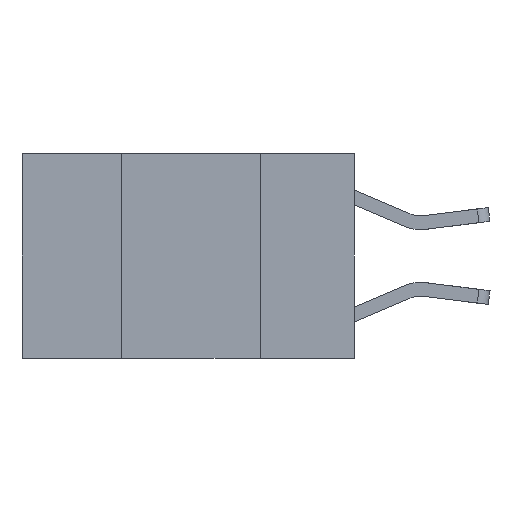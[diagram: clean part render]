
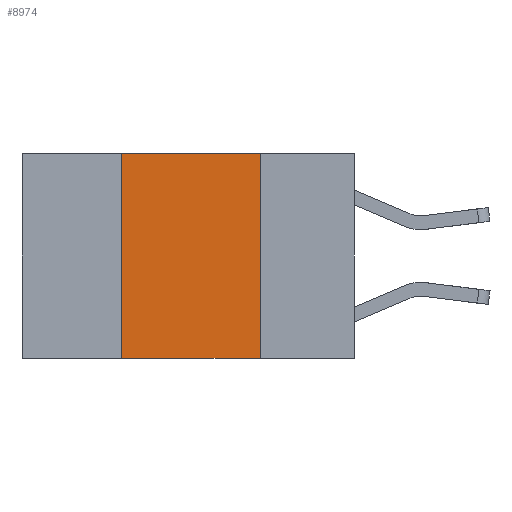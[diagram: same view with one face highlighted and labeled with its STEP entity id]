
A CAD part, left-side view. The second image highlights one B-rep face of the part: STEP entity #8974.
In plain terms, the highlighted planar face has unit normal (-1, 0, 0).
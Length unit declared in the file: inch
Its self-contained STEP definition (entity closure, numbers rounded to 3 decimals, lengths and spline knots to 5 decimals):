
#59 = VERTEX_POINT ( 'NONE', #8099 ) ;
#444 = CARTESIAN_POINT ( 'NONE',  ( 0., 0.42, 0. ) ) ;
#585 = EDGE_LOOP ( 'NONE', ( #4037, #6360, #8165, #7606 ) ) ;
#648 = LINE ( 'NONE', #1263, #4809 ) ;
#688 = DIRECTION ( 'NONE',  ( 0., -1., 0. ) ) ;
#1263 = CARTESIAN_POINT ( 'NONE',  ( 0., 0.17, 0. ) ) ;
#1276 = DIRECTION ( 'NONE',  ( 0., 0., -1. ) ) ;
#1296 = EDGE_CURVE ( 'NONE', #3190, #59, #648, .T. ) ;
#1344 = VERTEX_POINT ( 'NONE', #444 ) ;
#1619 = DIRECTION ( 'NONE',  ( 0., 0., 1. ) ) ;
#1663 = DIRECTION ( 'NONE',  ( 1., 0., 0. ) ) ;
#2662 = LINE ( 'NONE', #5832, #8879 ) ;
#3190 = VERTEX_POINT ( 'NONE', #5365 ) ;
#3290 = CARTESIAN_POINT ( 'NONE',  ( 0., 0.42, 0. ) ) ;
#4037 = ORIENTED_EDGE ( 'NONE', *, *, #1296, .F. ) ;
#4129 = PLANE ( 'NONE',  #4927 ) ;
#4809 = VECTOR ( 'NONE', #1276, 39.37008 ) ;
#4863 = CARTESIAN_POINT ( 'NONE',  ( 0., 0.6, 0. ) ) ;
#4927 = AXIS2_PLACEMENT_3D ( 'NONE', #6601, #1663, #7398 ) ;
#5365 = CARTESIAN_POINT ( 'NONE',  ( 0., 0.17, 0. ) ) ;
#5819 = VECTOR ( 'NONE', #1619, 39.37008 ) ;
#5832 = CARTESIAN_POINT ( 'NONE',  ( 0., 0.6, -0.37 ) ) ;
#6015 = VERTEX_POINT ( 'NONE', #6807 ) ;
#6019 = VECTOR ( 'NONE', #688, 39.37008 ) ;
#6278 = LINE ( 'NONE', #4863, #6019 ) ;
#6360 = ORIENTED_EDGE ( 'NONE', *, *, #10103, .F. ) ;
#6362 = EDGE_CURVE ( 'NONE', #6015, #1344, #9731, .T. ) ;
#6601 = CARTESIAN_POINT ( 'NONE',  ( 0., 0.6, 0. ) ) ;
#6807 = CARTESIAN_POINT ( 'NONE',  ( 0., 0.42, -0.37 ) ) ;
#7398 = DIRECTION ( 'NONE',  ( 0., 0., -1. ) ) ;
#7602 = EDGE_CURVE ( 'NONE', #6015, #59, #2662, .T. ) ;
#7606 = ORIENTED_EDGE ( 'NONE', *, *, #7602, .T. ) ;
#8099 = CARTESIAN_POINT ( 'NONE',  ( 0., 0.17, -0.37 ) ) ;
#8165 = ORIENTED_EDGE ( 'NONE', *, *, #6362, .F. ) ;
#8599 = FACE_OUTER_BOUND ( 'NONE', #585, .T. ) ;
#8879 = VECTOR ( 'NONE', #9726, 39.37008 ) ;
#8974 = ADVANCED_FACE ( 'NONE', ( #8599 ), #4129, .F. ) ;
#9726 = DIRECTION ( 'NONE',  ( 0., -1., 0. ) ) ;
#9731 = LINE ( 'NONE', #3290, #5819 ) ;
#10103 = EDGE_CURVE ( 'NONE', #1344, #3190, #6278, .T. ) ;
